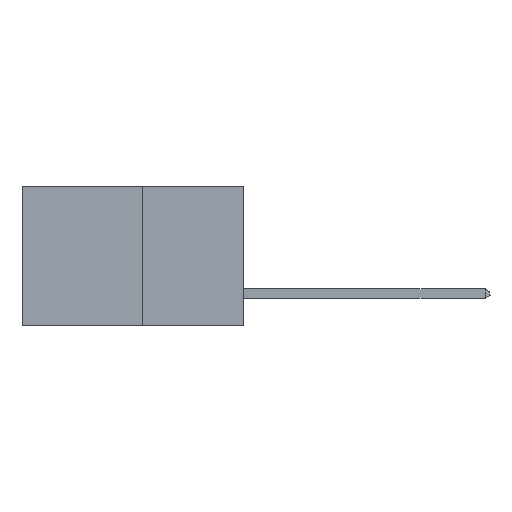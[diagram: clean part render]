
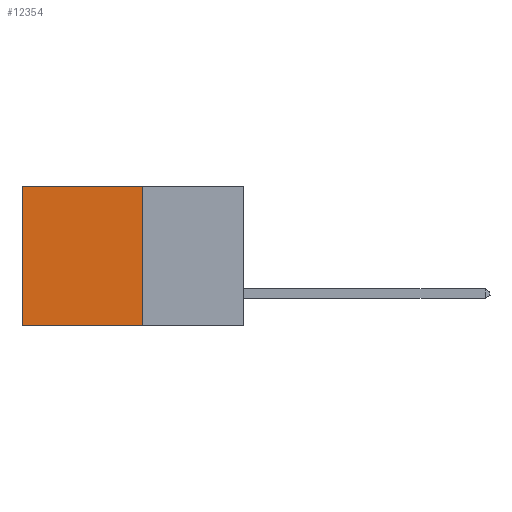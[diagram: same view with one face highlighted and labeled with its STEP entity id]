
A CAD part, left-side view. The second image highlights one B-rep face of the part: STEP entity #12354.
In plain terms, the highlighted planar face has unit normal (-1, 0, 0).
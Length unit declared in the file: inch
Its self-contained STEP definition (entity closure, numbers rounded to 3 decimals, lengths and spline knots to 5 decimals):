
#289 = CARTESIAN_POINT ( 'NONE',  ( 0.277, 0.27, -0.37 ) ) ;
#511 = ORIENTED_EDGE ( 'NONE', *, *, #6100, .T. ) ;
#661 = CARTESIAN_POINT ( 'NONE',  ( 0.277, 0.59, 0. ) ) ;
#1326 = LINE ( 'NONE', #4785, #10786 ) ;
#1492 = DIRECTION ( 'NONE',  ( 1., 0., 0. ) ) ;
#1714 = EDGE_CURVE ( 'NONE', #8403, #3817, #13394, .T. ) ;
#1864 = DIRECTION ( 'NONE',  ( 0., 1., 0. ) ) ;
#2142 = VERTEX_POINT ( 'NONE', #661 ) ;
#2550 = LINE ( 'NONE', #4634, #8566 ) ;
#3817 = VERTEX_POINT ( 'NONE', #4023 ) ;
#4001 = DIRECTION ( 'NONE',  ( 0., 0., -1. ) ) ;
#4023 = CARTESIAN_POINT ( 'NONE',  ( 0.277, 0.27, -0.37 ) ) ;
#4073 = CARTESIAN_POINT ( 'NONE',  ( 0.277, 0.27, 0. ) ) ;
#4634 = CARTESIAN_POINT ( 'NONE',  ( 0.277, 0.27, -0.37 ) ) ;
#4785 = CARTESIAN_POINT ( 'NONE',  ( 0.277, 0.59, -0.37 ) ) ;
#5880 = DIRECTION ( 'NONE',  ( 0., 1., 0. ) ) ;
#6100 = EDGE_CURVE ( 'NONE', #8403, #2142, #6955, .T. ) ;
#6486 = CARTESIAN_POINT ( 'NONE',  ( 0.277, 0.59, -0.37 ) ) ;
#6955 = LINE ( 'NONE', #10145, #10066 ) ;
#7171 = VERTEX_POINT ( 'NONE', #6486 ) ;
#7290 = ORIENTED_EDGE ( 'NONE', *, *, #1714, .F. ) ;
#7292 = VECTOR ( 'NONE', #4001, 39.37008 ) ;
#8049 = AXIS2_PLACEMENT_3D ( 'NONE', #289, #1492, #9802 ) ;
#8403 = VERTEX_POINT ( 'NONE', #4073 ) ;
#8566 = VECTOR ( 'NONE', #5880, 39.37008 ) ;
#8667 = PLANE ( 'NONE',  #8049 ) ;
#9142 = ORIENTED_EDGE ( 'NONE', *, *, #14638, .F. ) ;
#9784 = CARTESIAN_POINT ( 'NONE',  ( 0.277, 0.27, -0.37 ) ) ;
#9802 = DIRECTION ( 'NONE',  ( 0., 0., -1. ) ) ;
#10066 = VECTOR ( 'NONE', #1864, 39.37008 ) ;
#10145 = CARTESIAN_POINT ( 'NONE',  ( 0.277, 0.27, 0. ) ) ;
#10447 = EDGE_CURVE ( 'NONE', #2142, #7171, #1326, .T. ) ;
#10786 = VECTOR ( 'NONE', #13009, 39.37008 ) ;
#12354 = ADVANCED_FACE ( 'NONE', ( #14600 ), #8667, .F. ) ;
#12641 = EDGE_LOOP ( 'NONE', ( #13342, #9142, #7290, #511 ) ) ;
#13009 = DIRECTION ( 'NONE',  ( 0., 0., -1. ) ) ;
#13342 = ORIENTED_EDGE ( 'NONE', *, *, #10447, .T. ) ;
#13394 = LINE ( 'NONE', #9784, #7292 ) ;
#14600 = FACE_OUTER_BOUND ( 'NONE', #12641, .T. ) ;
#14638 = EDGE_CURVE ( 'NONE', #3817, #7171, #2550, .T. ) ;
